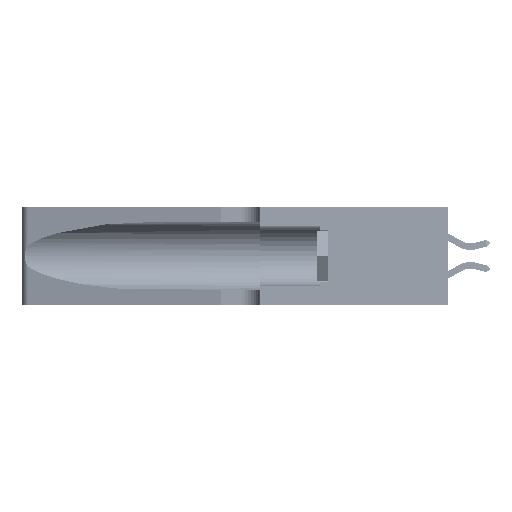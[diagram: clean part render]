
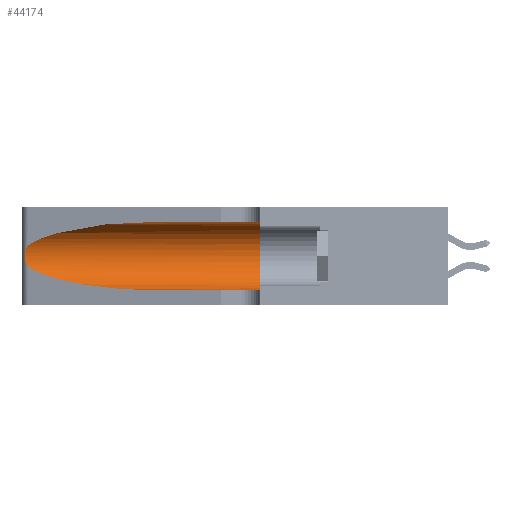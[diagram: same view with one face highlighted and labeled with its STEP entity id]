
A CAD part, left-side view. The second image highlights one B-rep face of the part: STEP entity #44174.
In plain terms, the highlighted cylindrical face has radius 3.308 mm (diameter 6.617 mm), a partial arc.
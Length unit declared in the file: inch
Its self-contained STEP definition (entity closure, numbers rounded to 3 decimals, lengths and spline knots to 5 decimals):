
#431 = VECTOR ( 'NONE', #44456, 39.37008 ) ;
#482 = EDGE_CURVE ( 'NONE', #25566, #32321, #20291, .T. ) ;
#492 = VERTEX_POINT ( 'NONE', #25326 ) ;
#720 = CARTESIAN_POINT ( 'NONE',  ( 0.2373, 1.15595, 0.08982 ) ) ;
#848 = EDGE_CURVE ( 'NONE', #25566, #3846, #45679, .T. ) ;
#1132 = FACE_OUTER_BOUND ( 'NONE', #28718, .T. ) ;
#2132 = EDGE_CURVE ( 'NONE', #492, #6980, #19544, .T. ) ;
#2392 = CARTESIAN_POINT ( 'NONE',  ( 0.1305, 1.61858, 0.31525 ) ) ;
#3409 = ORIENTED_EDGE ( 'NONE', *, *, #34282, .T. ) ;
#3846 = VERTEX_POINT ( 'NONE', #36044 ) ;
#4612 = CARTESIAN_POINT ( 'NONE',  ( 0.25787, 1.23484, 0.2124 ) ) ;
#6980 = VERTEX_POINT ( 'NONE', #8690 ) ;
#7295 = CARTESIAN_POINT ( 'NONE',  ( 0.25487, 1.22718, 0.22369 ) ) ;
#7930 = CARTESIAN_POINT ( 'NONE',  ( 0.1305, 0.35, 0.31525 ) ) ;
#8438 = CARTESIAN_POINT ( 'NONE',  ( 0.26018, 1.23835, 0.19895 ) ) ;
#8456 = CARTESIAN_POINT ( 'NONE',  ( 0.25487, 1.22718, 0.14631 ) ) ;
#8690 = CARTESIAN_POINT ( 'NONE',  ( 0.1305, 0.35, 0.05475 ) ) ;
#8972 = VERTEX_POINT ( 'NONE', #32810 ) ;
#10218 = VECTOR ( 'NONE', #21527, 39.37008 ) ;
#12256 = CARTESIAN_POINT ( 'NONE',  ( 0.26075, 1.23896, 0.178 ) ) ;
#12339 = DIRECTION ( 'NONE',  ( 0., 1., 0. ) ) ;
#16094 = CARTESIAN_POINT ( 'NONE',  ( 0.25856, 1.23593, 0.16098 ) ) ;
#16117 = CARTESIAN_POINT ( 'NONE',  ( 0.18966, 0.96281, 0.05475 ) ) ;
#18000 = AXIS2_PLACEMENT_3D ( 'NONE', #40472, #36659, #44267 ) ;
#19544 = LINE ( 'NONE', #33237, #431 ) ;
#19878 = CARTESIAN_POINT ( 'NONE',  ( 0.25639, 1.23186, 0.15144 ) ) ;
#20291 = LINE ( 'NONE', #2392, #10218 ) ;
#21527 = DIRECTION ( 'NONE',  ( 0., -1., 0. ) ) ;
#22741 = ORIENTED_EDGE ( 'NONE', *, *, #2132, .T. ) ;
#22804 = ORIENTED_EDGE ( 'NONE', *, *, #31183, .T. ) ;
#23703 = CARTESIAN_POINT ( 'NONE',  ( 0.25487, 1.22718, 0.14631 ) ) ;
#23798 = CYLINDRICAL_SURFACE ( 'NONE', #18000, 0.13025 ) ;
#25326 = CARTESIAN_POINT ( 'NONE',  ( 0.1305, 0.72297, 0.05475 ) ) ;
#25566 = VERTEX_POINT ( 'NONE', #42291 ) ;
#26236 = CARTESIAN_POINT ( 'NONE',  ( 0.18966, 0.96281, 0.31525 ) ) ;
#27352 = CARTESIAN_POINT ( 'NONE',  ( 0.25639, 1.23184, 0.21858 ) ) ;
#28718 = EDGE_LOOP ( 'NONE', ( #32206, #3409, #22804, #22741, #44127, #38660 ) ) ;
#29648 = B_SPLINE_CURVE_WITH_KNOTS ( 'NONE', 3,
 ( #34794, #46155, #27352, #4612, #31149, #8438, #34942, #12256, #38741, #16094, #42552, #19878, #46321, #23703 ),
 .UNSPECIFIED., .F., .F.,
 ( 4, 2, 2, 2, 2, 2, 4 ),
 ( 0., 0.00027, 0.00053, 0.00107, 0.0016, 0.00187, 0.00214 ),
 .UNSPECIFIED. ) ;
#30023 = CARTESIAN_POINT ( 'NONE',  ( 0.1305, 0.72297, 0.31525 ) ) ;
#31149 = CARTESIAN_POINT ( 'NONE',  ( 0.25854, 1.2359, 0.20912 ) ) ;
#31183 = EDGE_CURVE ( 'NONE', #8972, #492, #38422, .T. ) ;
#32206 = ORIENTED_EDGE ( 'NONE', *, *, #848, .T. ) ;
#32321 = VERTEX_POINT ( 'NONE', #7930 ) ;
#32810 = CARTESIAN_POINT ( 'NONE',  ( 0.25487, 1.22718, 0.14631 ) ) ;
#33237 = CARTESIAN_POINT ( 'NONE',  ( 0.1305, 1.61858, 0.05475 ) ) ;
#33378 = CIRCLE ( 'NONE', #37475, 0.13025 ) ;
#34282 = EDGE_CURVE ( 'NONE', #3846, #8972, #29648, .T. ) ;
#34794 = CARTESIAN_POINT ( 'NONE',  ( 0.25487, 1.22718, 0.22369 ) ) ;
#34942 = CARTESIAN_POINT ( 'NONE',  ( 0.26075, 1.23896, 0.19203 ) ) ;
#35037 = CARTESIAN_POINT ( 'NONE',  ( 0.1305, 0.35, 0.185 ) ) ;
#36044 = CARTESIAN_POINT ( 'NONE',  ( 0.25487, 1.22718, 0.22369 ) ) ;
#36659 = DIRECTION ( 'NONE',  ( 0., -1., 0. ) ) ;
#37475 = AXIS2_PLACEMENT_3D ( 'NONE', #35037, #12339, #38827 ) ;
#38422 =( BOUNDED_CURVE ( )  B_SPLINE_CURVE ( 3, ( #8456, #720, #16117, #42568 ),
 .UNSPECIFIED., .F., .F. ) 
 B_SPLINE_CURVE_WITH_KNOTS ( ( 4, 4 ),
 ( 3.44316, 4.71239 ),
 .UNSPECIFIED. ) 
 CURVE ( )  GEOMETRIC_REPRESENTATION_ITEM ( )  RATIONAL_B_SPLINE_CURVE ( ( 1., 0.87, 0.87, 1. ) ) 
 REPRESENTATION_ITEM ( '' )  );
#38660 = ORIENTED_EDGE ( 'NONE', *, *, #482, .F. ) ;
#38741 = CARTESIAN_POINT ( 'NONE',  ( 0.26017, 1.23833, 0.17102 ) ) ;
#38827 = DIRECTION ( 'NONE',  ( 0., 0., 1. ) ) ;
#39079 = EDGE_CURVE ( 'NONE', #32321, #6980, #33378, .T. ) ;
#40472 = CARTESIAN_POINT ( 'NONE',  ( 0.1305, 1.61858, 0.185 ) ) ;
#42291 = CARTESIAN_POINT ( 'NONE',  ( 0.1305, 0.72297, 0.31525 ) ) ;
#42552 = CARTESIAN_POINT ( 'NONE',  ( 0.25789, 1.23486, 0.15765 ) ) ;
#42568 = CARTESIAN_POINT ( 'NONE',  ( 0.1305, 0.72297, 0.05475 ) ) ;
#44127 = ORIENTED_EDGE ( 'NONE', *, *, #39079, .F. ) ;
#44174 = ADVANCED_FACE ( 'NONE', ( #1132 ), #23798, .F. ) ;
#44267 = DIRECTION ( 'NONE',  ( 0., 0., -1. ) ) ;
#44456 = DIRECTION ( 'NONE',  ( 0., -1., 0. ) ) ;
#45679 =( BOUNDED_CURVE ( )  B_SPLINE_CURVE ( 3, ( #30023, #26236, #48822, #7295 ),
 .UNSPECIFIED., .F., .F. ) 
 B_SPLINE_CURVE_WITH_KNOTS ( ( 4, 4 ),
 ( 1.5708, 2.84003 ),
 .UNSPECIFIED. ) 
 CURVE ( )  GEOMETRIC_REPRESENTATION_ITEM ( )  RATIONAL_B_SPLINE_CURVE ( ( 1., 0.87, 0.87, 1. ) ) 
 REPRESENTATION_ITEM ( '' )  );
#46155 = CARTESIAN_POINT ( 'NONE',  ( 0.25555, 1.22994, 0.2215 ) ) ;
#46321 = CARTESIAN_POINT ( 'NONE',  ( 0.25555, 1.22993, 0.14849 ) ) ;
#48822 = CARTESIAN_POINT ( 'NONE',  ( 0.2373, 1.15595, 0.28018 ) ) ;
